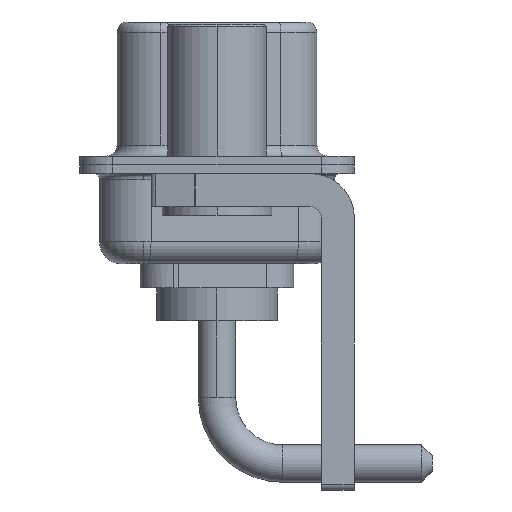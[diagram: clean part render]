
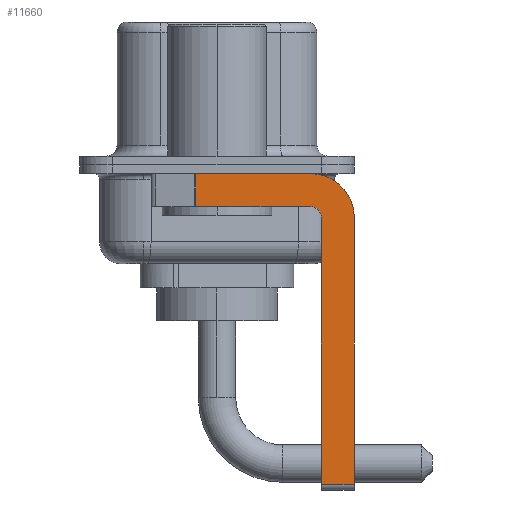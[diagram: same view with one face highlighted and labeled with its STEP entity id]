
A CAD part, left-side view. The second image highlights one B-rep face of the part: STEP entity #11660.
In plain terms, the highlighted planar face has unit normal (-1, 0, 0).
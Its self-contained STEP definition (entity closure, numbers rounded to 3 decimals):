
#84 = DIRECTION ( 'NONE',  ( 0., 0., 1. ) ) ;
#208 = ORIENTED_EDGE ( 'NONE', *, *, #18020, .F. ) ;
#248 = VERTEX_POINT ( 'NONE', #1124 ) ;
#1124 = CARTESIAN_POINT ( 'NONE',  ( -2.9, -6.25, -14.55 ) ) ;
#1231 = LINE ( 'NONE', #12573, #12380 ) ;
#1298 = VERTEX_POINT ( 'NONE', #16541 ) ;
#1658 = EDGE_LOOP ( 'NONE', ( #3258, #8530, #11701, #14322, #208, #10526, #7876, #6894 ) ) ;
#1825 = CARTESIAN_POINT ( 'NONE',  ( -2.9, -4.25, -2.4 ) ) ;
#1873 = CARTESIAN_POINT ( 'NONE',  ( -2.9, 0.978, -1.9 ) ) ;
#1959 = DIRECTION ( 'NONE',  ( 1., 0., 0. ) ) ;
#2269 = EDGE_CURVE ( 'NONE', #8411, #3365, #4284, .T. ) ;
#2320 = LINE ( 'NONE', #8050, #9660 ) ;
#3258 = ORIENTED_EDGE ( 'NONE', *, *, #8123, .F. ) ;
#3365 = VERTEX_POINT ( 'NONE', #12265 ) ;
#3404 = EDGE_CURVE ( 'NONE', #13222, #7788, #13131, .T. ) ;
#4161 = CARTESIAN_POINT ( 'NONE',  ( -2.9, -6.25, -2.4 ) ) ;
#4284 = CIRCLE ( 'NONE', #9022, 0.5 ) ;
#5373 = LINE ( 'NONE', #5724, #9148 ) ;
#5724 = CARTESIAN_POINT ( 'NONE',  ( -2.9, 3., -0.4 ) ) ;
#6073 = PLANE ( 'NONE',  #17752 ) ;
#6894 = ORIENTED_EDGE ( 'NONE', *, *, #9722, .F. ) ;
#7510 = DIRECTION ( 'NONE',  ( 0., 0., -1. ) ) ;
#7563 = DIRECTION ( 'NONE',  ( 0., 0., -1. ) ) ;
#7587 = DIRECTION ( 'NONE',  ( 0., 0., -1. ) ) ;
#7788 = VERTEX_POINT ( 'NONE', #13840 ) ;
#7831 = VECTOR ( 'NONE', #8570, 1000. ) ;
#7876 = ORIENTED_EDGE ( 'NONE', *, *, #14963, .F. ) ;
#8050 = CARTESIAN_POINT ( 'NONE',  ( -2.9, -4.25, -14.55 ) ) ;
#8123 = EDGE_CURVE ( 'NONE', #13222, #12126, #5373, .T. ) ;
#8155 = EDGE_CURVE ( 'NONE', #3365, #7788, #1231, .T. ) ;
#8370 = CARTESIAN_POINT ( 'NONE',  ( -2.9, 0.978, -0.4 ) ) ;
#8411 = VERTEX_POINT ( 'NONE', #16125 ) ;
#8530 = ORIENTED_EDGE ( 'NONE', *, *, #3404, .T. ) ;
#8570 = DIRECTION ( 'NONE',  ( 0., 0., -1. ) ) ;
#9022 = AXIS2_PLACEMENT_3D ( 'NONE', #1825, #14081, #84 ) ;
#9148 = VECTOR ( 'NONE', #12662, 1000. ) ;
#9641 = VECTOR ( 'NONE', #7510, 1000. ) ;
#9660 = VECTOR ( 'NONE', #17868, 1000. ) ;
#9722 = EDGE_CURVE ( 'NONE', #12126, #9986, #14462, .T. ) ;
#9986 = VERTEX_POINT ( 'NONE', #4161 ) ;
#10351 = AXIS2_PLACEMENT_3D ( 'NONE', #11543, #1959, #7587 ) ;
#10414 = DIRECTION ( 'NONE',  ( 1., 0., 0. ) ) ;
#10526 = ORIENTED_EDGE ( 'NONE', *, *, #16016, .T. ) ;
#11543 = CARTESIAN_POINT ( 'NONE',  ( -2.9, -4.25, -2.4 ) ) ;
#11660 = ADVANCED_FACE ( 'NONE', ( #11696 ), #6073, .F. ) ;
#11696 = FACE_OUTER_BOUND ( 'NONE', #1658, .T. ) ;
#11701 = ORIENTED_EDGE ( 'NONE', *, *, #8155, .F. ) ;
#12126 = VERTEX_POINT ( 'NONE', #17188 ) ;
#12265 = CARTESIAN_POINT ( 'NONE',  ( -2.9, -4.25, -1.9 ) ) ;
#12380 = VECTOR ( 'NONE', #12746, 1000. ) ;
#12573 = CARTESIAN_POINT ( 'NONE',  ( -2.9, -4.25, -1.9 ) ) ;
#12662 = DIRECTION ( 'NONE',  ( 0., -1., 0. ) ) ;
#12746 = DIRECTION ( 'NONE',  ( 0., 1., 0. ) ) ;
#13131 = LINE ( 'NONE', #1873, #9641 ) ;
#13220 = LINE ( 'NONE', #14682, #16453 ) ;
#13222 = VERTEX_POINT ( 'NONE', #8370 ) ;
#13840 = CARTESIAN_POINT ( 'NONE',  ( -2.9, 0.978, -1.9 ) ) ;
#14081 = DIRECTION ( 'NONE',  ( -1., 0., 0. ) ) ;
#14322 = ORIENTED_EDGE ( 'NONE', *, *, #2269, .F. ) ;
#14462 = CIRCLE ( 'NONE', #10351, 2. ) ;
#14554 = CARTESIAN_POINT ( 'NONE',  ( -2.9, -4.25, -2.4 ) ) ;
#14682 = CARTESIAN_POINT ( 'NONE',  ( -2.9, -4.75, -14.8 ) ) ;
#14963 = EDGE_CURVE ( 'NONE', #9986, #248, #16919, .T. ) ;
#15545 = CARTESIAN_POINT ( 'NONE',  ( -2.9, -6.25, -2.4 ) ) ;
#16016 = EDGE_CURVE ( 'NONE', #1298, #248, #2320, .T. ) ;
#16049 = DIRECTION ( 'NONE',  ( 0., 0., 1. ) ) ;
#16125 = CARTESIAN_POINT ( 'NONE',  ( -2.9, -4.75, -2.4 ) ) ;
#16453 = VECTOR ( 'NONE', #16049, 1000. ) ;
#16541 = CARTESIAN_POINT ( 'NONE',  ( -2.9, -4.75, -14.55 ) ) ;
#16919 = LINE ( 'NONE', #15545, #7831 ) ;
#17188 = CARTESIAN_POINT ( 'NONE',  ( -2.9, -4.25, -0.4 ) ) ;
#17752 = AXIS2_PLACEMENT_3D ( 'NONE', #14554, #10414, #7563 ) ;
#17868 = DIRECTION ( 'NONE',  ( 0., -1., 0. ) ) ;
#18020 = EDGE_CURVE ( 'NONE', #1298, #8411, #13220, .T. ) ;
